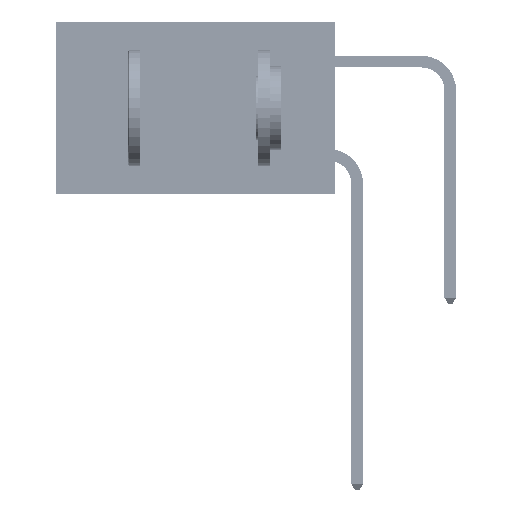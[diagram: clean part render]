
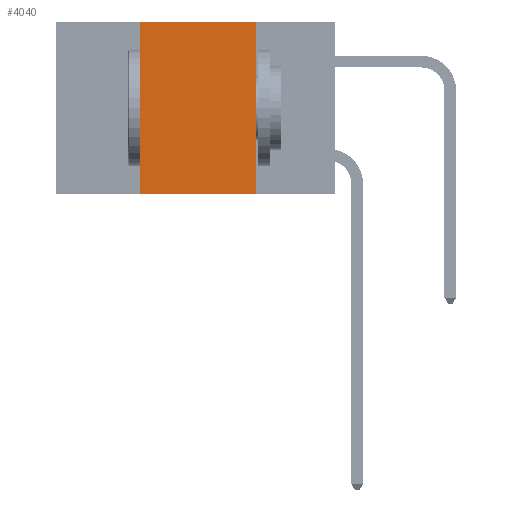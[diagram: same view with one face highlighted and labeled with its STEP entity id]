
A CAD part, left-side view. The second image highlights one B-rep face of the part: STEP entity #4040.
In plain terms, the highlighted planar face has unit normal (-1, 0, 0).
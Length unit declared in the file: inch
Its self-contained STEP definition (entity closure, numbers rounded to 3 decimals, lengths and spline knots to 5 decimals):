
#60 = DIRECTION ( 'NONE',  ( 0., -1., 0. ) ) ;
#228 = CARTESIAN_POINT ( 'NONE',  ( 0., 0.17, -0.37 ) ) ;
#2110 = VECTOR ( 'NONE', #17773, 39.37008 ) ;
#2198 = VECTOR ( 'NONE', #4293, 39.37008 ) ;
#2475 = ORIENTED_EDGE ( 'NONE', *, *, #35300, .F. ) ;
#4040 = ADVANCED_FACE ( 'NONE', ( #18185 ), #42792, .F. ) ;
#4288 = VECTOR ( 'NONE', #60, 39.37008 ) ;
#4293 = DIRECTION ( 'NONE',  ( 0., 0., 1. ) ) ;
#6888 = CARTESIAN_POINT ( 'NONE',  ( 0., 0.6, 0. ) ) ;
#7666 = CARTESIAN_POINT ( 'NONE',  ( 0., 0.42, -0.37 ) ) ;
#7975 = CARTESIAN_POINT ( 'NONE',  ( 0., 0.17, 0. ) ) ;
#10118 = ORIENTED_EDGE ( 'NONE', *, *, #16018, .T. ) ;
#14125 = CARTESIAN_POINT ( 'NONE',  ( 0., 0.17, 0. ) ) ;
#14446 = VERTEX_POINT ( 'NONE', #7975 ) ;
#16018 = EDGE_CURVE ( 'NONE', #19124, #30660, #38158, .T. ) ;
#16366 = LINE ( 'NONE', #40263, #2198 ) ;
#17773 = DIRECTION ( 'NONE',  ( 0., 0., -1. ) ) ;
#17927 = EDGE_CURVE ( 'NONE', #19124, #29095, #16366, .T. ) ;
#18185 = FACE_OUTER_BOUND ( 'NONE', #42868, .T. ) ;
#18495 = LINE ( 'NONE', #6888, #4288 ) ;
#19124 = VERTEX_POINT ( 'NONE', #7666 ) ;
#24616 = CARTESIAN_POINT ( 'NONE',  ( 0., 0.6, 0. ) ) ;
#29095 = VERTEX_POINT ( 'NONE', #43643 ) ;
#30660 = VERTEX_POINT ( 'NONE', #228 ) ;
#31827 = CARTESIAN_POINT ( 'NONE',  ( 0., 0.6, -0.37 ) ) ;
#31835 = ORIENTED_EDGE ( 'NONE', *, *, #33872, .F. ) ;
#33872 = EDGE_CURVE ( 'NONE', #14446, #30660, #44775, .T. ) ;
#34900 = ORIENTED_EDGE ( 'NONE', *, *, #17927, .F. ) ;
#35300 = EDGE_CURVE ( 'NONE', #29095, #14446, #18495, .T. ) ;
#38158 = LINE ( 'NONE', #31827, #45541 ) ;
#40263 = CARTESIAN_POINT ( 'NONE',  ( 0., 0.42, 0. ) ) ;
#40847 = AXIS2_PLACEMENT_3D ( 'NONE', #24616, #42948, #46137 ) ;
#42792 = PLANE ( 'NONE',  #40847 ) ;
#42868 = EDGE_LOOP ( 'NONE', ( #31835, #2475, #34900, #10118 ) ) ;
#42948 = DIRECTION ( 'NONE',  ( 1., 0., 0. ) ) ;
#43010 = DIRECTION ( 'NONE',  ( 0., -1., 0. ) ) ;
#43643 = CARTESIAN_POINT ( 'NONE',  ( 0., 0.42, 0. ) ) ;
#44775 = LINE ( 'NONE', #14125, #2110 ) ;
#45541 = VECTOR ( 'NONE', #43010, 39.37008 ) ;
#46137 = DIRECTION ( 'NONE',  ( 0., 0., -1. ) ) ;
